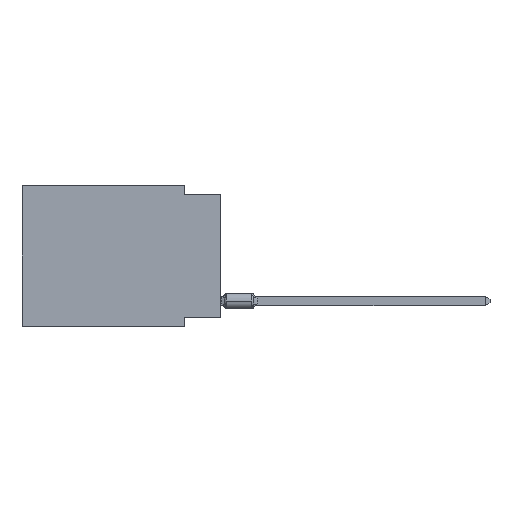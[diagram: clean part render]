
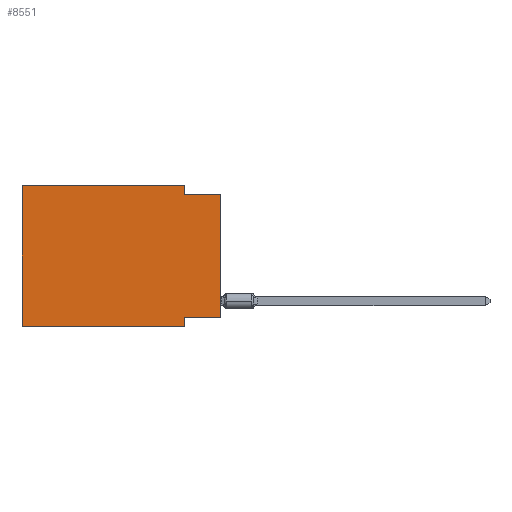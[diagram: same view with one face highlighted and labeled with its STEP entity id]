
A CAD part, left-side view. The second image highlights one B-rep face of the part: STEP entity #8551.
In plain terms, the highlighted planar face has unit normal (-1, 0, 0).
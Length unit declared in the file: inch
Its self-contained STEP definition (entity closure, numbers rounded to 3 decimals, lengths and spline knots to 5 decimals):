
#269 = CARTESIAN_POINT ( 'NONE',  ( 0., 0.55, 0. ) ) ;
#778 = EDGE_CURVE ( 'NONE', #27789, #16087, #9351, .T. ) ;
#1432 = VECTOR ( 'NONE', #24933, 39.37008 ) ;
#1560 = LINE ( 'NONE', #8361, #28326 ) ;
#2622 = DIRECTION ( 'NONE',  ( 1., 0., 0. ) ) ;
#2707 = LINE ( 'NONE', #11461, #23069 ) ;
#3473 = DIRECTION ( 'NONE',  ( 0., -1., 0. ) ) ;
#3573 = DIRECTION ( 'NONE',  ( 0., 0., -1. ) ) ;
#4355 = VERTEX_POINT ( 'NONE', #25158 ) ;
#4416 = ORIENTED_EDGE ( 'NONE', *, *, #9070, .F. ) ;
#4837 = FACE_OUTER_BOUND ( 'NONE', #6170, .T. ) ;
#4925 = CARTESIAN_POINT ( 'NONE',  ( 0., 0.1, -0.025 ) ) ;
#5229 = DIRECTION ( 'NONE',  ( 0., -1., 0. ) ) ;
#5240 = CARTESIAN_POINT ( 'NONE',  ( 0., 0.55, 0. ) ) ;
#5740 = DIRECTION ( 'NONE',  ( 0., 0., -1. ) ) ;
#6108 = ORIENTED_EDGE ( 'NONE', *, *, #778, .T. ) ;
#6170 = EDGE_LOOP ( 'NONE', ( #6108, #4416, #25452, #15072, #21304, #7730, #11143, #22124 ) ) ;
#6185 = EDGE_CURVE ( 'NONE', #8117, #15831, #2707, .T. ) ;
#6253 = CARTESIAN_POINT ( 'NONE',  ( 0., 0.1, -0.39 ) ) ;
#6323 = CARTESIAN_POINT ( 'NONE',  ( 0., 0.1, 0. ) ) ;
#7276 = DIRECTION ( 'NONE',  ( 0., 0., 1. ) ) ;
#7423 = CARTESIAN_POINT ( 'NONE',  ( 0., 0., 0. ) ) ;
#7454 = DIRECTION ( 'NONE',  ( 0., 0., 1. ) ) ;
#7730 = ORIENTED_EDGE ( 'NONE', *, *, #6185, .T. ) ;
#8095 = AXIS2_PLACEMENT_3D ( 'NONE', #269, #2622, #13880 ) ;
#8117 = VERTEX_POINT ( 'NONE', #25143 ) ;
#8361 = CARTESIAN_POINT ( 'NONE',  ( 0., 0.55, 0. ) ) ;
#8447 = CARTESIAN_POINT ( 'NONE',  ( 0., 0., -0.025 ) ) ;
#8551 = ADVANCED_FACE ( 'NONE', ( #4837 ), #27038, .F. ) ;
#9070 = EDGE_CURVE ( 'NONE', #25401, #16087, #10371, .T. ) ;
#9351 = LINE ( 'NONE', #7423, #26881 ) ;
#10371 = LINE ( 'NONE', #8447, #16638 ) ;
#10421 = EDGE_CURVE ( 'NONE', #17959, #15831, #26063, .T. ) ;
#11143 = ORIENTED_EDGE ( 'NONE', *, *, #10421, .F. ) ;
#11461 = CARTESIAN_POINT ( 'NONE',  ( 0., 0.55, -0.39 ) ) ;
#12806 = VECTOR ( 'NONE', #7454, 39.37008 ) ;
#12886 = EDGE_CURVE ( 'NONE', #4355, #24084, #1560, .T. ) ;
#13865 = CARTESIAN_POINT ( 'NONE',  ( 0., 0., -0.365 ) ) ;
#13880 = DIRECTION ( 'NONE',  ( 0., 0., -1. ) ) ;
#14916 = CARTESIAN_POINT ( 'NONE',  ( 0., 0.1, 0. ) ) ;
#15072 = ORIENTED_EDGE ( 'NONE', *, *, #12886, .F. ) ;
#15831 = VERTEX_POINT ( 'NONE', #6253 ) ;
#16087 = VERTEX_POINT ( 'NONE', #25414 ) ;
#16178 = EDGE_CURVE ( 'NONE', #24084, #25401, #19788, .T. ) ;
#16202 = CARTESIAN_POINT ( 'NONE',  ( 0., 0., -0.365 ) ) ;
#16286 = EDGE_CURVE ( 'NONE', #27789, #17959, #20220, .T. ) ;
#16480 = LINE ( 'NONE', #5240, #12806 ) ;
#16638 = VECTOR ( 'NONE', #19393, 39.37008 ) ;
#17746 = CARTESIAN_POINT ( 'NONE',  ( 0., 0.1, -0.365 ) ) ;
#17959 = VERTEX_POINT ( 'NONE', #17746 ) ;
#19393 = DIRECTION ( 'NONE',  ( 0., -1., 0. ) ) ;
#19788 = LINE ( 'NONE', #14916, #25523 ) ;
#20220 = LINE ( 'NONE', #13865, #1432 ) ;
#21304 = ORIENTED_EDGE ( 'NONE', *, *, #27915, .F. ) ;
#22124 = ORIENTED_EDGE ( 'NONE', *, *, #16286, .F. ) ;
#23069 = VECTOR ( 'NONE', #5229, 39.37008 ) ;
#23983 = CARTESIAN_POINT ( 'NONE',  ( 0., 0.1, -0.39 ) ) ;
#24084 = VERTEX_POINT ( 'NONE', #6323 ) ;
#24933 = DIRECTION ( 'NONE',  ( 0., 1., 0. ) ) ;
#25143 = CARTESIAN_POINT ( 'NONE',  ( 0., 0.55, -0.39 ) ) ;
#25158 = CARTESIAN_POINT ( 'NONE',  ( 0., 0.55, 0. ) ) ;
#25401 = VERTEX_POINT ( 'NONE', #4925 ) ;
#25414 = CARTESIAN_POINT ( 'NONE',  ( 0., 0., -0.025 ) ) ;
#25452 = ORIENTED_EDGE ( 'NONE', *, *, #16178, .F. ) ;
#25519 = VECTOR ( 'NONE', #3573, 39.37008 ) ;
#25523 = VECTOR ( 'NONE', #5740, 39.37008 ) ;
#26063 = LINE ( 'NONE', #23983, #25519 ) ;
#26881 = VECTOR ( 'NONE', #7276, 39.37008 ) ;
#27038 = PLANE ( 'NONE',  #8095 ) ;
#27789 = VERTEX_POINT ( 'NONE', #16202 ) ;
#27915 = EDGE_CURVE ( 'NONE', #8117, #4355, #16480, .T. ) ;
#28326 = VECTOR ( 'NONE', #3473, 39.37008 ) ;
